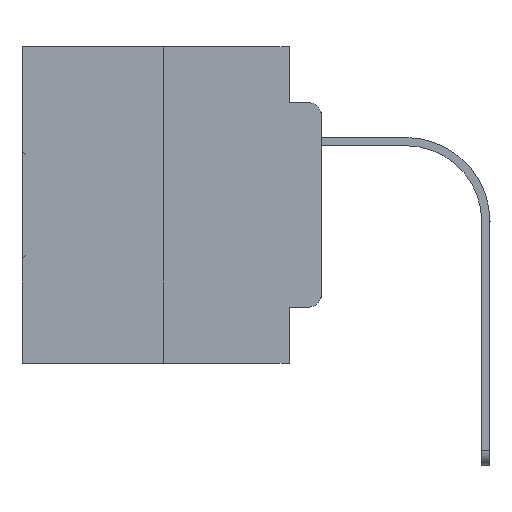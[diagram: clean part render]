
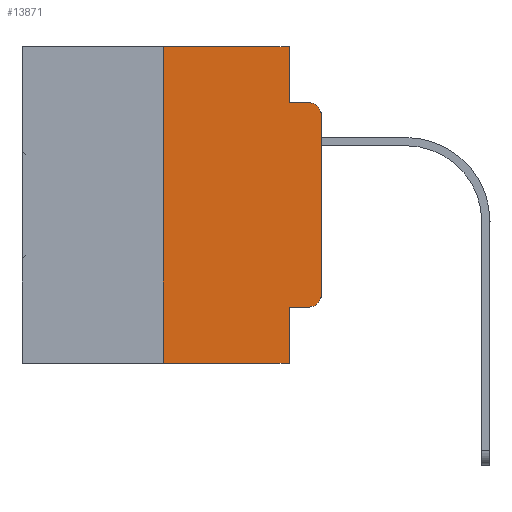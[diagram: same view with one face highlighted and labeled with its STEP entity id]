
A CAD part, left-side view. The second image highlights one B-rep face of the part: STEP entity #13871.
In plain terms, the highlighted planar face has unit normal (-1, 0, 0).
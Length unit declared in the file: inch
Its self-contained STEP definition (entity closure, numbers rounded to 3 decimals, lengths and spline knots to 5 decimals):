
#122 = CARTESIAN_POINT ( 'NONE',  ( 0., 0.051, -0.4115 ) ) ;
#124 = EDGE_CURVE ( 'NONE', #2036, #3616, #4669, .T. ) ;
#1868 = CARTESIAN_POINT ( 'NONE',  ( 0., 0.25, 0. ) ) ;
#1963 = VERTEX_POINT ( 'NONE', #19738 ) ;
#2031 = LINE ( 'NONE', #11563, #15593 ) ;
#2036 = VERTEX_POINT ( 'NONE', #5354 ) ;
#2124 = LINE ( 'NONE', #18718, #30019 ) ;
#2379 = ORIENTED_EDGE ( 'NONE', *, *, #24446, .T. ) ;
#2474 = DIRECTION ( 'NONE',  ( 0., 0., 1. ) ) ;
#2695 = FACE_OUTER_BOUND ( 'NONE', #24771, .T. ) ;
#2992 = VECTOR ( 'NONE', #2474, 39.37008 ) ;
#3140 = CARTESIAN_POINT ( 'NONE',  ( 0., 0.051, -0.0885 ) ) ;
#3528 = DIRECTION ( 'NONE',  ( 0., 0., -1. ) ) ;
#3616 = VERTEX_POINT ( 'NONE', #26324 ) ;
#4276 = ORIENTED_EDGE ( 'NONE', *, *, #13009, .F. ) ;
#4669 = LINE ( 'NONE', #30982, #25829 ) ;
#5098 = CARTESIAN_POINT ( 'NONE',  ( 0., 0.25, -0.5 ) ) ;
#5251 = EDGE_CURVE ( 'NONE', #1963, #15827, #21418, .T. ) ;
#5342 = VERTEX_POINT ( 'NONE', #14509 ) ;
#5354 = CARTESIAN_POINT ( 'NONE',  ( 0., 0., -0.3915 ) ) ;
#5981 = CARTESIAN_POINT ( 'NONE',  ( 0., 0.051, -0.0885 ) ) ;
#6273 = ORIENTED_EDGE ( 'NONE', *, *, #23238, .F. ) ;
#6454 = VERTEX_POINT ( 'NONE', #13040 ) ;
#6941 = ORIENTED_EDGE ( 'NONE', *, *, #7430, .T. ) ;
#7396 = DIRECTION ( 'NONE',  ( 0., 0., -1. ) ) ;
#7430 = EDGE_CURVE ( 'NONE', #24133, #15055, #2124, .T. ) ;
#7549 = DIRECTION ( 'NONE',  ( 1., 0., 0. ) ) ;
#7674 = LINE ( 'NONE', #3140, #12064 ) ;
#8571 = DIRECTION ( 'NONE',  ( -1., 0., 0. ) ) ;
#9691 = VERTEX_POINT ( 'NONE', #5981 ) ;
#9900 = PLANE ( 'NONE',  #17615 ) ;
#10058 = CARTESIAN_POINT ( 'NONE',  ( 0., 0.473, 0. ) ) ;
#11178 = CARTESIAN_POINT ( 'NONE',  ( 0., 0.02, -0.1085 ) ) ;
#11563 = CARTESIAN_POINT ( 'NONE',  ( 0., 0.473, 0. ) ) ;
#11772 = ORIENTED_EDGE ( 'NONE', *, *, #28493, .F. ) ;
#12008 = DIRECTION ( 'NONE',  ( 0., -1., 0. ) ) ;
#12064 = VECTOR ( 'NONE', #12348, 39.37008 ) ;
#12348 = DIRECTION ( 'NONE',  ( 0., -1., 0. ) ) ;
#12394 = AXIS2_PLACEMENT_3D ( 'NONE', #20458, #8571, #15443 ) ;
#12648 = EDGE_CURVE ( 'NONE', #9691, #5342, #7674, .T. ) ;
#13009 = EDGE_CURVE ( 'NONE', #6454, #21367, #2031, .T. ) ;
#13040 = CARTESIAN_POINT ( 'NONE',  ( 0., 0.25, 0. ) ) ;
#13335 = VECTOR ( 'NONE', #24083, 39.37008 ) ;
#13871 = ADVANCED_FACE ( 'NONE', ( #2695 ), #9900, .F. ) ;
#14327 = EDGE_CURVE ( 'NONE', #15827, #2036, #25955, .T. ) ;
#14509 = CARTESIAN_POINT ( 'NONE',  ( 0., 0.02, -0.0885 ) ) ;
#15055 = VERTEX_POINT ( 'NONE', #21959 ) ;
#15406 = CARTESIAN_POINT ( 'NONE',  ( 0., 0.051, 0. ) ) ;
#15443 = DIRECTION ( 'NONE',  ( 0., 0., -1. ) ) ;
#15446 = CARTESIAN_POINT ( 'NONE',  ( 0., 0.051, 0. ) ) ;
#15593 = VECTOR ( 'NONE', #12008, 39.37008 ) ;
#15827 = VERTEX_POINT ( 'NONE', #29401 ) ;
#16051 = VECTOR ( 'NONE', #3528, 39.37008 ) ;
#17615 = AXIS2_PLACEMENT_3D ( 'NONE', #10058, #7549, #19433 ) ;
#18394 = DIRECTION ( 'NONE',  ( -1., 0., 0. ) ) ;
#18625 = AXIS2_PLACEMENT_3D ( 'NONE', #11178, #18394, #7396 ) ;
#18718 = CARTESIAN_POINT ( 'NONE',  ( 0., 0.473, -0.5 ) ) ;
#19433 = DIRECTION ( 'NONE',  ( 0., 0., -1. ) ) ;
#19588 = ORIENTED_EDGE ( 'NONE', *, *, #124, .T. ) ;
#19738 = CARTESIAN_POINT ( 'NONE',  ( 0., 0.051, -0.4115 ) ) ;
#20458 = CARTESIAN_POINT ( 'NONE',  ( 0., 0.02, -0.3915 ) ) ;
#20822 = LINE ( 'NONE', #28676, #22721 ) ;
#21076 = EDGE_CURVE ( 'NONE', #24133, #6454, #23773, .T. ) ;
#21367 = VERTEX_POINT ( 'NONE', #15446 ) ;
#21418 = LINE ( 'NONE', #122, #13335 ) ;
#21888 = DIRECTION ( 'NONE',  ( 0., 0., -1. ) ) ;
#21959 = CARTESIAN_POINT ( 'NONE',  ( 0., 0.051, -0.5 ) ) ;
#22721 = VECTOR ( 'NONE', #21888, 39.37008 ) ;
#23238 = EDGE_CURVE ( 'NONE', #1963, #15055, #27671, .T. ) ;
#23456 = DIRECTION ( 'NONE',  ( 0., 0., 1. ) ) ;
#23773 = LINE ( 'NONE', #1868, #2992 ) ;
#24083 = DIRECTION ( 'NONE',  ( 0., -1., 0. ) ) ;
#24133 = VERTEX_POINT ( 'NONE', #5098 ) ;
#24446 = EDGE_CURVE ( 'NONE', #3616, #5342, #24633, .T. ) ;
#24633 = CIRCLE ( 'NONE', #18625, 0.02 ) ;
#24771 = EDGE_LOOP ( 'NONE', ( #19588, #2379, #28617, #11772, #4276, #29060, #6941, #6273, #28435, #25047 ) ) ;
#25047 = ORIENTED_EDGE ( 'NONE', *, *, #14327, .T. ) ;
#25829 = VECTOR ( 'NONE', #23456, 39.37008 ) ;
#25955 = CIRCLE ( 'NONE', #12394, 0.02 ) ;
#26324 = CARTESIAN_POINT ( 'NONE',  ( 0., 0., -0.1085 ) ) ;
#27671 = LINE ( 'NONE', #15406, #16051 ) ;
#28435 = ORIENTED_EDGE ( 'NONE', *, *, #5251, .T. ) ;
#28493 = EDGE_CURVE ( 'NONE', #21367, #9691, #20822, .T. ) ;
#28617 = ORIENTED_EDGE ( 'NONE', *, *, #12648, .F. ) ;
#28676 = CARTESIAN_POINT ( 'NONE',  ( 0., 0.051, 0. ) ) ;
#28752 = DIRECTION ( 'NONE',  ( 0., -1., 0. ) ) ;
#29060 = ORIENTED_EDGE ( 'NONE', *, *, #21076, .F. ) ;
#29401 = CARTESIAN_POINT ( 'NONE',  ( 0., 0.02, -0.4115 ) ) ;
#30019 = VECTOR ( 'NONE', #28752, 39.37008 ) ;
#30982 = CARTESIAN_POINT ( 'NONE',  ( 0., 0., 0. ) ) ;
